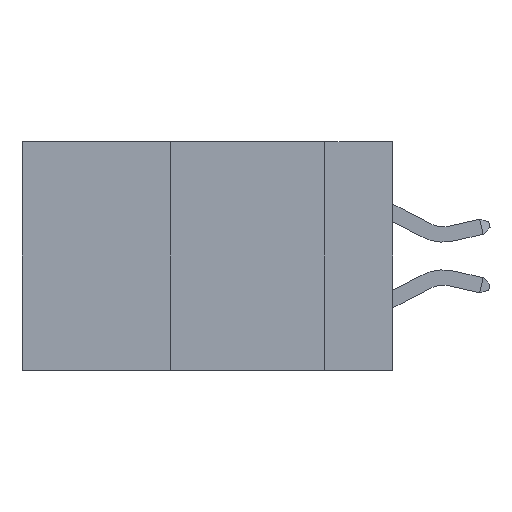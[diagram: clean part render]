
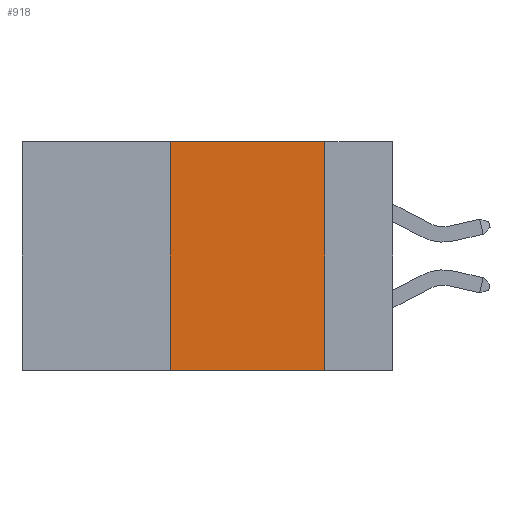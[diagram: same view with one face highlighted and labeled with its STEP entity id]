
A CAD part, left-side view. The second image highlights one B-rep face of the part: STEP entity #918.
In plain terms, the highlighted planar face has unit normal (-1, 0, 0).
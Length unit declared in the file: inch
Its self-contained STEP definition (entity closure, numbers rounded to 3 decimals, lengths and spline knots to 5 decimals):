
#264 = ORIENTED_EDGE ( 'NONE', *, *, #5533, .T. ) ;
#472 = DIRECTION ( 'NONE',  ( 0., 0., -1. ) ) ;
#756 = VECTOR ( 'NONE', #10605, 39.37008 ) ;
#918 = ADVANCED_FACE ( 'NONE', ( #12122 ), #4174, .F. ) ;
#1396 = CARTESIAN_POINT ( 'NONE',  ( 0., 0.11, 0. ) ) ;
#1462 = EDGE_CURVE ( 'NONE', #9092, #11231, #12023, .T. ) ;
#1910 = CARTESIAN_POINT ( 'NONE',  ( 0., 0.11, -0.37 ) ) ;
#2011 = DIRECTION ( 'NONE',  ( 1., 0., 0. ) ) ;
#2020 = ORIENTED_EDGE ( 'NONE', *, *, #12311, .F. ) ;
#3077 = DIRECTION ( 'NONE',  ( 0., 0., -1. ) ) ;
#3597 = LINE ( 'NONE', #6178, #6930 ) ;
#3813 = EDGE_LOOP ( 'NONE', ( #2020, #8048, #7295, #264 ) ) ;
#4174 = PLANE ( 'NONE',  #7886 ) ;
#4297 = VECTOR ( 'NONE', #472, 39.37008 ) ;
#5533 = EDGE_CURVE ( 'NONE', #9092, #13143, #12728, .T. ) ;
#5718 = CARTESIAN_POINT ( 'NONE',  ( 0., 0.36, -0.37 ) ) ;
#6178 = CARTESIAN_POINT ( 'NONE',  ( 0., 0.6, 0. ) ) ;
#6521 = CARTESIAN_POINT ( 'NONE',  ( 0., 0.11, 0. ) ) ;
#6930 = VECTOR ( 'NONE', #10349, 39.37008 ) ;
#7036 = CARTESIAN_POINT ( 'NONE',  ( 0., 0.36, 0. ) ) ;
#7295 = ORIENTED_EDGE ( 'NONE', *, *, #1462, .F. ) ;
#7886 = AXIS2_PLACEMENT_3D ( 'NONE', #11261, #2011, #3077 ) ;
#8048 = ORIENTED_EDGE ( 'NONE', *, *, #8295, .F. ) ;
#8295 = EDGE_CURVE ( 'NONE', #11231, #8444, #3597, .T. ) ;
#8444 = VERTEX_POINT ( 'NONE', #6521 ) ;
#8923 = CARTESIAN_POINT ( 'NONE',  ( 0., 0.36, 0. ) ) ;
#9092 = VERTEX_POINT ( 'NONE', #5718 ) ;
#9585 = CARTESIAN_POINT ( 'NONE',  ( 0., 0.6, -0.37 ) ) ;
#10349 = DIRECTION ( 'NONE',  ( 0., -1., 0. ) ) ;
#10605 = DIRECTION ( 'NONE',  ( 0., -1., 0. ) ) ;
#10875 = VECTOR ( 'NONE', #10937, 39.37008 ) ;
#10937 = DIRECTION ( 'NONE',  ( 0., 0., 1. ) ) ;
#11231 = VERTEX_POINT ( 'NONE', #8923 ) ;
#11261 = CARTESIAN_POINT ( 'NONE',  ( 0., 0.6, 0. ) ) ;
#11432 = LINE ( 'NONE', #1396, #4297 ) ;
#12023 = LINE ( 'NONE', #7036, #10875 ) ;
#12122 = FACE_OUTER_BOUND ( 'NONE', #3813, .T. ) ;
#12311 = EDGE_CURVE ( 'NONE', #8444, #13143, #11432, .T. ) ;
#12728 = LINE ( 'NONE', #9585, #756 ) ;
#13143 = VERTEX_POINT ( 'NONE', #1910 ) ;
